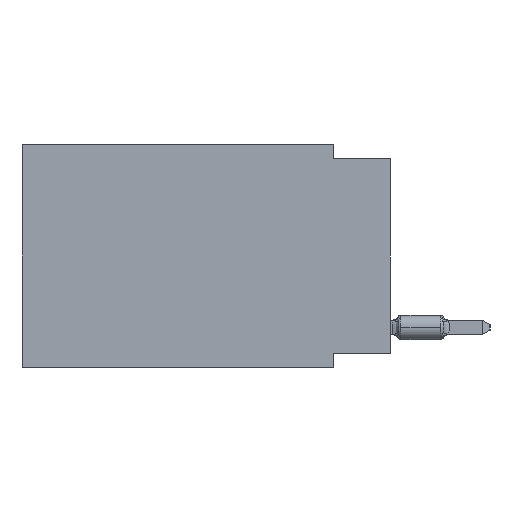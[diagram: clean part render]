
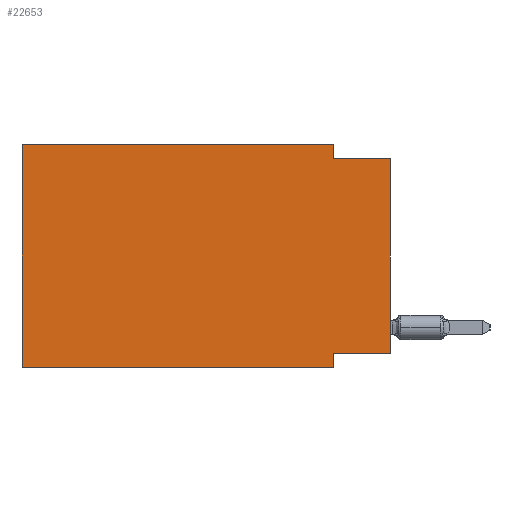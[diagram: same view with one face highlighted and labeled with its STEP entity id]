
A CAD part, left-side view. The second image highlights one B-rep face of the part: STEP entity #22653.
In plain terms, the highlighted planar face has unit normal (-1, 0, 0).
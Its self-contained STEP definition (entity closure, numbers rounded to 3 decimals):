
#5392 = AXIS2_PLACEMENT_3D ( 'NONE', #46829, #51330, #42033 ) ;
#5869 = CARTESIAN_POINT ( 'NONE',  ( 0., 0., -0.635 ) ) ;
#7157 = VERTEX_POINT ( 'NONE', #37109 ) ;
#7796 = VERTEX_POINT ( 'NONE', #13287 ) ;
#8440 = VERTEX_POINT ( 'NONE', #26256 ) ;
#9382 = VERTEX_POINT ( 'NONE', #23313 ) ;
#10338 = VECTOR ( 'NONE', #54172, 1000. ) ;
#10357 = LINE ( 'NONE', #5869, #13331 ) ;
#10819 = VERTEX_POINT ( 'NONE', #22433 ) ;
#13142 = VERTEX_POINT ( 'NONE', #18581 ) ;
#13287 = CARTESIAN_POINT ( 'NONE',  ( 0., 16.383, -9.906 ) ) ;
#13331 = VECTOR ( 'NONE', #42171, 1000. ) ;
#13879 = VERTEX_POINT ( 'NONE', #55548 ) ;
#13888 = ORIENTED_EDGE ( 'NONE', *, *, #20151, .F. ) ;
#16041 = ORIENTED_EDGE ( 'NONE', *, *, #49907, .F. ) ;
#16091 = CARTESIAN_POINT ( 'NONE',  ( 0., 2.54, 0. ) ) ;
#16538 = VECTOR ( 'NONE', #48520, 1000. ) ;
#16705 = CARTESIAN_POINT ( 'NONE',  ( 0., 2.54, -9.906 ) ) ;
#18581 = CARTESIAN_POINT ( 'NONE',  ( 0., 0., -0.635 ) ) ;
#18857 = DIRECTION ( 'NONE',  ( 0., 0., 1. ) ) ;
#20151 = EDGE_CURVE ( 'NONE', #8440, #7157, #39232, .T. ) ;
#21470 = LINE ( 'NONE', #16091, #26247 ) ;
#22433 = CARTESIAN_POINT ( 'NONE',  ( 0., 16.383, 0. ) ) ;
#22551 = VECTOR ( 'NONE', #42540, 1000. ) ;
#22653 = ADVANCED_FACE ( 'NONE', ( #37536 ), #24035, .F. ) ;
#22672 = CARTESIAN_POINT ( 'NONE',  ( 0., 16.383, 0. ) ) ;
#23262 = CARTESIAN_POINT ( 'NONE',  ( 0., 16.383, 0. ) ) ;
#23313 = CARTESIAN_POINT ( 'NONE',  ( 0., 2.54, -0.635 ) ) ;
#23971 = CARTESIAN_POINT ( 'NONE',  ( 0., 0., 0. ) ) ;
#24035 = PLANE ( 'NONE',  #5392 ) ;
#24197 = ORIENTED_EDGE ( 'NONE', *, *, #35891, .F. ) ;
#24235 = LINE ( 'NONE', #56028, #22551 ) ;
#26247 = VECTOR ( 'NONE', #57503, 1000. ) ;
#26256 = CARTESIAN_POINT ( 'NONE',  ( 0., 2.54, -9.271 ) ) ;
#26727 = VECTOR ( 'NONE', #27464, 1000. ) ;
#27464 = DIRECTION ( 'NONE',  ( 0., -1., 0. ) ) ;
#29786 = ORIENTED_EDGE ( 'NONE', *, *, #41855, .F. ) ;
#35596 = CARTESIAN_POINT ( 'NONE',  ( 0., 0., -9.271 ) ) ;
#35891 = EDGE_CURVE ( 'NONE', #13879, #9382, #21470, .T. ) ;
#36757 = ORIENTED_EDGE ( 'NONE', *, *, #56161, .T. ) ;
#37109 = CARTESIAN_POINT ( 'NONE',  ( 0., 2.54, -9.906 ) ) ;
#37536 = FACE_OUTER_BOUND ( 'NONE', #46258, .T. ) ;
#38286 = LINE ( 'NONE', #23971, #52480 ) ;
#39232 = LINE ( 'NONE', #16705, #16538 ) ;
#40382 = EDGE_CURVE ( 'NONE', #10819, #13879, #55354, .T. ) ;
#40408 = LINE ( 'NONE', #35596, #45067 ) ;
#41528 = ORIENTED_EDGE ( 'NONE', *, *, #51092, .F. ) ;
#41855 = EDGE_CURVE ( 'NONE', #45081, #8440, #40408, .T. ) ;
#42033 = DIRECTION ( 'NONE',  ( 0., 0., -1. ) ) ;
#42171 = DIRECTION ( 'NONE',  ( 0., -1., 0. ) ) ;
#42540 = DIRECTION ( 'NONE',  ( 0., -1., 0. ) ) ;
#44501 = CARTESIAN_POINT ( 'NONE',  ( 0., 0., -9.271 ) ) ;
#45067 = VECTOR ( 'NONE', #53603, 1000. ) ;
#45081 = VERTEX_POINT ( 'NONE', #44501 ) ;
#46258 = EDGE_LOOP ( 'NONE', ( #36757, #41528, #24197, #47603, #16041, #48794, #13888, #29786 ) ) ;
#46829 = CARTESIAN_POINT ( 'NONE',  ( 0., 16.383, 0. ) ) ;
#47371 = EDGE_CURVE ( 'NONE', #7796, #7157, #24235, .T. ) ;
#47603 = ORIENTED_EDGE ( 'NONE', *, *, #40382, .F. ) ;
#48520 = DIRECTION ( 'NONE',  ( 0., 0., -1. ) ) ;
#48794 = ORIENTED_EDGE ( 'NONE', *, *, #47371, .T. ) ;
#49907 = EDGE_CURVE ( 'NONE', #7796, #10819, #54780, .T. ) ;
#51092 = EDGE_CURVE ( 'NONE', #9382, #13142, #10357, .T. ) ;
#51330 = DIRECTION ( 'NONE',  ( 1., 0., 0. ) ) ;
#52480 = VECTOR ( 'NONE', #18857, 1000. ) ;
#53603 = DIRECTION ( 'NONE',  ( 0., 1., 0. ) ) ;
#54172 = DIRECTION ( 'NONE',  ( 0., 0., 1. ) ) ;
#54780 = LINE ( 'NONE', #22672, #10338 ) ;
#55354 = LINE ( 'NONE', #23262, #26727 ) ;
#55548 = CARTESIAN_POINT ( 'NONE',  ( 0., 2.54, 0. ) ) ;
#56028 = CARTESIAN_POINT ( 'NONE',  ( 0., 16.383, -9.906 ) ) ;
#56161 = EDGE_CURVE ( 'NONE', #45081, #13142, #38286, .T. ) ;
#57503 = DIRECTION ( 'NONE',  ( 0., 0., -1. ) ) ;
